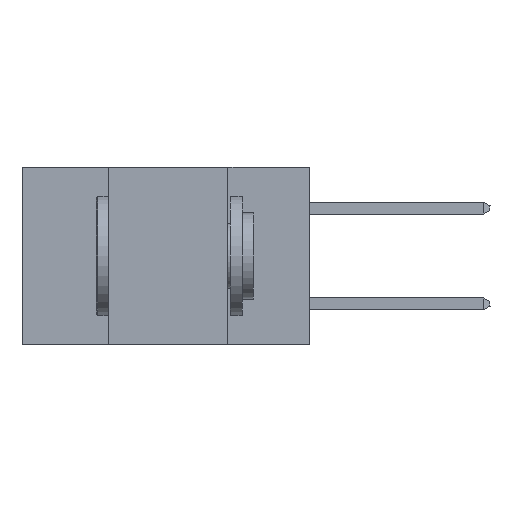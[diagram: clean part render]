
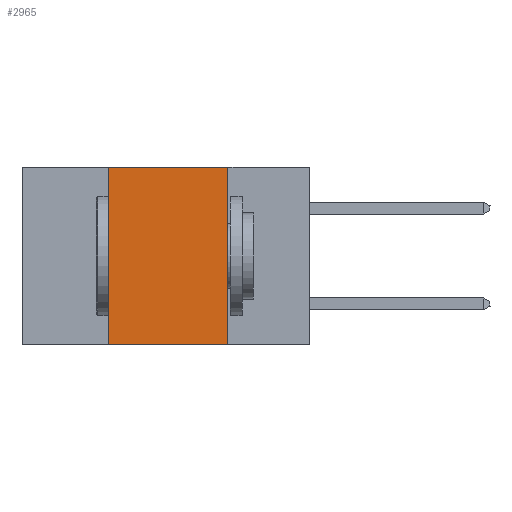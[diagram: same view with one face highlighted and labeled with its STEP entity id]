
A CAD part, left-side view. The second image highlights one B-rep face of the part: STEP entity #2965.
In plain terms, the highlighted planar face has unit normal (-1, 0, 0).
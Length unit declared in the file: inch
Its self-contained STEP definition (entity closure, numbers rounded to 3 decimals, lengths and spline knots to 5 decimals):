
#962 = DIRECTION ( 'NONE',  ( 0., 0., 1. ) ) ;
#1279 = VECTOR ( 'NONE', #18195, 39.37008 ) ;
#1814 = LINE ( 'NONE', #7154, #15101 ) ;
#2107 = LINE ( 'NONE', #30872, #1279 ) ;
#2327 = VERTEX_POINT ( 'NONE', #27148 ) ;
#2481 = CARTESIAN_POINT ( 'NONE',  ( 0., 0.17, 0. ) ) ;
#2965 = ADVANCED_FACE ( 'NONE', ( #3377 ), #12081, .F. ) ;
#3377 = FACE_OUTER_BOUND ( 'NONE', #24678, .T. ) ;
#6528 = EDGE_CURVE ( 'NONE', #2327, #22796, #2107, .T. ) ;
#6735 = CARTESIAN_POINT ( 'NONE',  ( 0., 0.6, 0. ) ) ;
#7154 = CARTESIAN_POINT ( 'NONE',  ( 0., 0.6, 0. ) ) ;
#7524 = CARTESIAN_POINT ( 'NONE',  ( 0., 0.42, 0. ) ) ;
#9139 = ORIENTED_EDGE ( 'NONE', *, *, #26204, .F. ) ;
#11601 = CARTESIAN_POINT ( 'NONE',  ( 0., 0.17, 0. ) ) ;
#11625 = CARTESIAN_POINT ( 'NONE',  ( 0., 0.42, 0. ) ) ;
#12081 = PLANE ( 'NONE',  #21807 ) ;
#12558 = VECTOR ( 'NONE', #23511, 39.37008 ) ;
#12613 = EDGE_CURVE ( 'NONE', #29859, #26454, #1814, .T. ) ;
#14672 = DIRECTION ( 'NONE',  ( 1., 0., 0. ) ) ;
#15101 = VECTOR ( 'NONE', #22813, 39.37008 ) ;
#16491 = ORIENTED_EDGE ( 'NONE', *, *, #29166, .F. ) ;
#18195 = DIRECTION ( 'NONE',  ( 0., -1., 0. ) ) ;
#18203 = VECTOR ( 'NONE', #962, 39.37008 ) ;
#19822 = ORIENTED_EDGE ( 'NONE', *, *, #6528, .T. ) ;
#20912 = ORIENTED_EDGE ( 'NONE', *, *, #12613, .F. ) ;
#20985 = CARTESIAN_POINT ( 'NONE',  ( 0., 0.17, -0.37 ) ) ;
#21048 = LINE ( 'NONE', #2481, #12558 ) ;
#21807 = AXIS2_PLACEMENT_3D ( 'NONE', #6735, #14672, #32660 ) ;
#22796 = VERTEX_POINT ( 'NONE', #20985 ) ;
#22813 = DIRECTION ( 'NONE',  ( 0., -1., 0. ) ) ;
#23511 = DIRECTION ( 'NONE',  ( 0., 0., -1. ) ) ;
#24678 = EDGE_LOOP ( 'NONE', ( #9139, #20912, #16491, #19822 ) ) ;
#26204 = EDGE_CURVE ( 'NONE', #26454, #22796, #21048, .T. ) ;
#26454 = VERTEX_POINT ( 'NONE', #11601 ) ;
#27148 = CARTESIAN_POINT ( 'NONE',  ( 0., 0.42, -0.37 ) ) ;
#29166 = EDGE_CURVE ( 'NONE', #2327, #29859, #31858, .T. ) ;
#29859 = VERTEX_POINT ( 'NONE', #7524 ) ;
#30872 = CARTESIAN_POINT ( 'NONE',  ( 0., 0.6, -0.37 ) ) ;
#31858 = LINE ( 'NONE', #11625, #18203 ) ;
#32660 = DIRECTION ( 'NONE',  ( 0., 0., -1. ) ) ;
